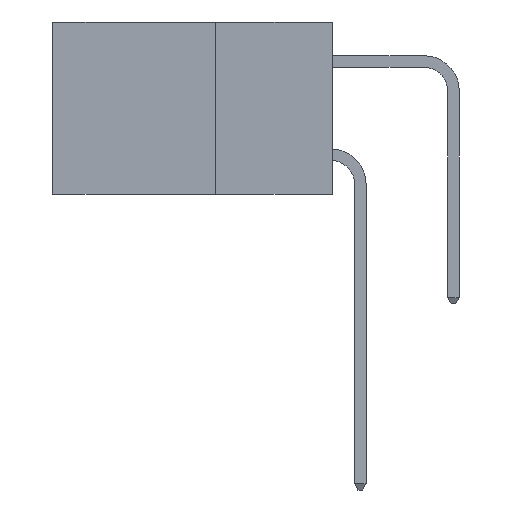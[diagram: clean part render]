
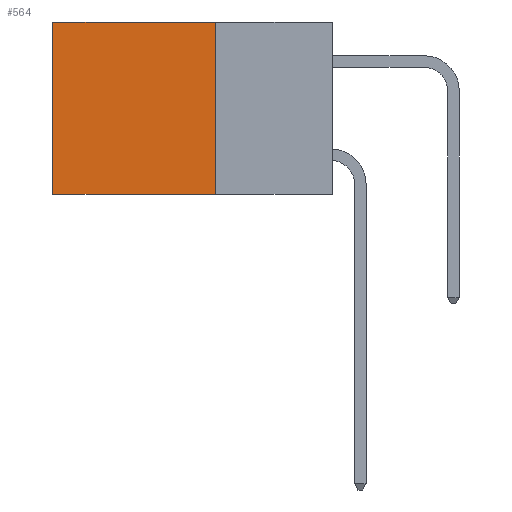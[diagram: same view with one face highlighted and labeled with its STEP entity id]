
A CAD part, left-side view. The second image highlights one B-rep face of the part: STEP entity #564.
In plain terms, the highlighted planar face has unit normal (-1, 0, 0).
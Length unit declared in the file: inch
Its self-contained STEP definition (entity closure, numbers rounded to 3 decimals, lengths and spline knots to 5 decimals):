
#285 = VECTOR ( 'NONE', #8598, 39.37008 ) ;
#564 = ADVANCED_FACE ( 'NONE', ( #2072 ), #6451, .F. ) ;
#612 = LINE ( 'NONE', #9106, #766 ) ;
#766 = VECTOR ( 'NONE', #7204, 39.37008 ) ;
#911 = DIRECTION ( 'NONE',  ( 1., 0., 0. ) ) ;
#1055 = CARTESIAN_POINT ( 'NONE',  ( 0.2615, 0.25, 0. ) ) ;
#1168 = VECTOR ( 'NONE', #5219, 39.37008 ) ;
#1540 = ORIENTED_EDGE ( 'NONE', *, *, #9298, .F. ) ;
#1718 = ORIENTED_EDGE ( 'NONE', *, *, #2147, .T. ) ;
#1755 = VERTEX_POINT ( 'NONE', #2722 ) ;
#1803 = ORIENTED_EDGE ( 'NONE', *, *, #2471, .F. ) ;
#2072 = FACE_OUTER_BOUND ( 'NONE', #2942, .T. ) ;
#2147 = EDGE_CURVE ( 'NONE', #10693, #1755, #612, .T. ) ;
#2173 = CARTESIAN_POINT ( 'NONE',  ( 0.2615, 0.25, -0.37 ) ) ;
#2471 = EDGE_CURVE ( 'NONE', #5943, #1755, #8930, .T. ) ;
#2722 = CARTESIAN_POINT ( 'NONE',  ( 0.2615, 0.6, -0.37 ) ) ;
#2942 = EDGE_LOOP ( 'NONE', ( #1718, #1803, #1540, #3665 ) ) ;
#3665 = ORIENTED_EDGE ( 'NONE', *, *, #10727, .T. ) ;
#3870 = VERTEX_POINT ( 'NONE', #1055 ) ;
#4659 = AXIS2_PLACEMENT_3D ( 'NONE', #7378, #911, #7335 ) ;
#5021 = LINE ( 'NONE', #2173, #285 ) ;
#5066 = CARTESIAN_POINT ( 'NONE',  ( 0.2615, 0.6, 0. ) ) ;
#5219 = DIRECTION ( 'NONE',  ( 0., 1., 0. ) ) ;
#5943 = VERTEX_POINT ( 'NONE', #10143 ) ;
#6110 = VECTOR ( 'NONE', #6930, 39.37008 ) ;
#6451 = PLANE ( 'NONE',  #4659 ) ;
#6930 = DIRECTION ( 'NONE',  ( 0., 1., 0. ) ) ;
#7006 = CARTESIAN_POINT ( 'NONE',  ( 0.2615, 0.25, -0.37 ) ) ;
#7204 = DIRECTION ( 'NONE',  ( 0., 0., -1. ) ) ;
#7335 = DIRECTION ( 'NONE',  ( 0., 0., -1. ) ) ;
#7378 = CARTESIAN_POINT ( 'NONE',  ( 0.2615, 0.25, -0.37 ) ) ;
#7546 = LINE ( 'NONE', #9735, #6110 ) ;
#8598 = DIRECTION ( 'NONE',  ( 0., 0., -1. ) ) ;
#8930 = LINE ( 'NONE', #7006, #1168 ) ;
#9106 = CARTESIAN_POINT ( 'NONE',  ( 0.2615, 0.6, -0.37 ) ) ;
#9298 = EDGE_CURVE ( 'NONE', #3870, #5943, #5021, .T. ) ;
#9735 = CARTESIAN_POINT ( 'NONE',  ( 0.2615, 0.25, 0. ) ) ;
#10143 = CARTESIAN_POINT ( 'NONE',  ( 0.2615, 0.25, -0.37 ) ) ;
#10693 = VERTEX_POINT ( 'NONE', #5066 ) ;
#10727 = EDGE_CURVE ( 'NONE', #3870, #10693, #7546, .T. ) ;
